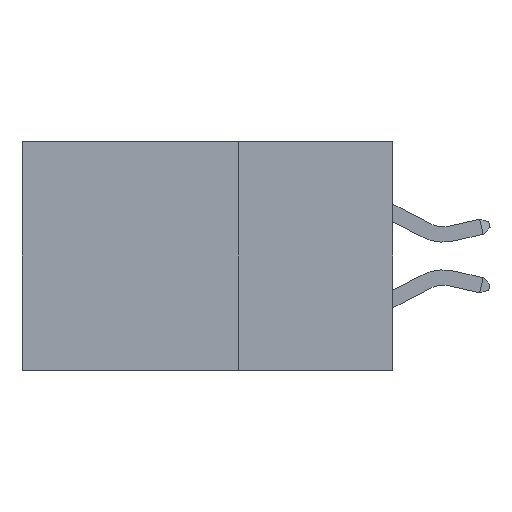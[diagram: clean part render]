
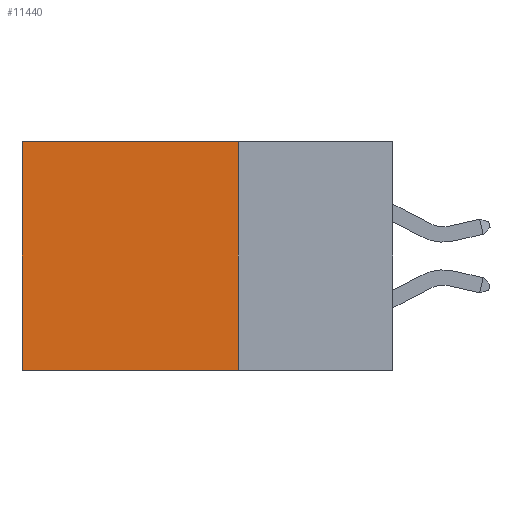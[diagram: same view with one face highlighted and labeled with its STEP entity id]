
A CAD part, left-side view. The second image highlights one B-rep face of the part: STEP entity #11440.
In plain terms, the highlighted planar face has unit normal (-1, 0, 0).
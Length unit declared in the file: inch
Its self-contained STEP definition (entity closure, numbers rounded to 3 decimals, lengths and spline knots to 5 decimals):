
#213 = VECTOR ( 'NONE', #10211, 39.37008 ) ;
#459 = VECTOR ( 'NONE', #3295, 39.37008 ) ;
#550 = VECTOR ( 'NONE', #1913, 39.37008 ) ;
#1390 = VERTEX_POINT ( 'NONE', #3018 ) ;
#1913 = DIRECTION ( 'NONE',  ( 0., 1., 0. ) ) ;
#1981 = DIRECTION ( 'NONE',  ( 0., 0., -1. ) ) ;
#2091 = CARTESIAN_POINT ( 'NONE',  ( 0.2875, 0.25, 0. ) ) ;
#2366 = EDGE_CURVE ( 'NONE', #1390, #6487, #4846, .T. ) ;
#2697 = LINE ( 'NONE', #11658, #459 ) ;
#3018 = CARTESIAN_POINT ( 'NONE',  ( 0.2875, 0.25, -0.37 ) ) ;
#3137 = PLANE ( 'NONE',  #5857 ) ;
#3295 = DIRECTION ( 'NONE',  ( 0., 1., 0. ) ) ;
#3633 = FACE_OUTER_BOUND ( 'NONE', #5759, .T. ) ;
#4076 = CARTESIAN_POINT ( 'NONE',  ( 0.2875, 0.25, 0. ) ) ;
#4193 = EDGE_CURVE ( 'NONE', #9444, #9381, #2697, .T. ) ;
#4260 = ORIENTED_EDGE ( 'NONE', *, *, #4193, .T. ) ;
#4522 = CARTESIAN_POINT ( 'NONE',  ( 0.2875, 0.6, 0. ) ) ;
#4846 = LINE ( 'NONE', #8564, #550 ) ;
#4946 = LINE ( 'NONE', #4522, #213 ) ;
#5759 = EDGE_LOOP ( 'NONE', ( #6008, #6277, #11726, #4260 ) ) ;
#5857 = AXIS2_PLACEMENT_3D ( 'NONE', #4076, #11648, #5985 ) ;
#5985 = DIRECTION ( 'NONE',  ( 0., 0., -1. ) ) ;
#6008 = ORIENTED_EDGE ( 'NONE', *, *, #11891, .T. ) ;
#6277 = ORIENTED_EDGE ( 'NONE', *, *, #2366, .F. ) ;
#6476 = LINE ( 'NONE', #2091, #10054 ) ;
#6487 = VERTEX_POINT ( 'NONE', #9448 ) ;
#8564 = CARTESIAN_POINT ( 'NONE',  ( 0.2875, 0.25, -0.37 ) ) ;
#8740 = CARTESIAN_POINT ( 'NONE',  ( 0.2875, 0.6, 0. ) ) ;
#9381 = VERTEX_POINT ( 'NONE', #8740 ) ;
#9444 = VERTEX_POINT ( 'NONE', #11805 ) ;
#9448 = CARTESIAN_POINT ( 'NONE',  ( 0.2875, 0.6, -0.37 ) ) ;
#10054 = VECTOR ( 'NONE', #1981, 39.37008 ) ;
#10055 = EDGE_CURVE ( 'NONE', #9444, #1390, #6476, .T. ) ;
#10211 = DIRECTION ( 'NONE',  ( 0., 0., -1. ) ) ;
#11440 = ADVANCED_FACE ( 'NONE', ( #3633 ), #3137, .F. ) ;
#11648 = DIRECTION ( 'NONE',  ( 1., 0., 0. ) ) ;
#11658 = CARTESIAN_POINT ( 'NONE',  ( 0.2875, 0.25, 0. ) ) ;
#11726 = ORIENTED_EDGE ( 'NONE', *, *, #10055, .F. ) ;
#11805 = CARTESIAN_POINT ( 'NONE',  ( 0.2875, 0.25, 0. ) ) ;
#11891 = EDGE_CURVE ( 'NONE', #9381, #6487, #4946, .T. ) ;
